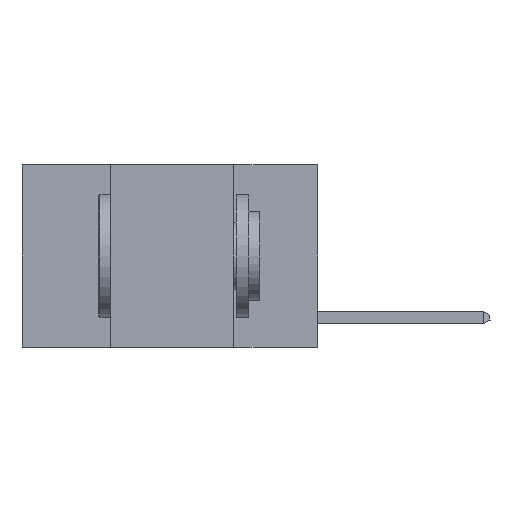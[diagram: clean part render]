
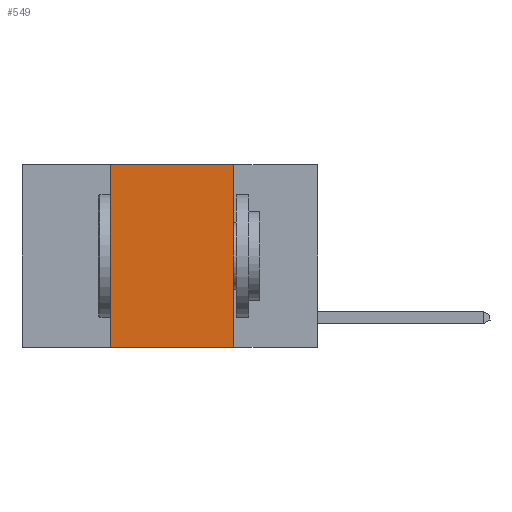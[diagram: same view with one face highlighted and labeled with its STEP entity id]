
A CAD part, left-side view. The second image highlights one B-rep face of the part: STEP entity #549.
In plain terms, the highlighted planar face has unit normal (-1, 0, 0).
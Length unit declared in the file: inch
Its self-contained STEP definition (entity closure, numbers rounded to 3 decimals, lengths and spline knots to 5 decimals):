
#181 = PLANE ( 'NONE',  #1054 ) ;
#549 = ADVANCED_FACE ( 'NONE', ( #6727 ), #181, .F. ) ;
#836 = ORIENTED_EDGE ( 'NONE', *, *, #5112, .F. ) ;
#945 = DIRECTION ( 'NONE',  ( 0., -1., 0. ) ) ;
#1054 = AXIS2_PLACEMENT_3D ( 'NONE', #6978, #3947, #5356 ) ;
#1161 = CARTESIAN_POINT ( 'NONE',  ( 0., 0.42, 0. ) ) ;
#2320 = CARTESIAN_POINT ( 'NONE',  ( 0., 0.17, 0. ) ) ;
#2432 = EDGE_LOOP ( 'NONE', ( #836, #7963, #5006, #6387 ) ) ;
#2466 = CARTESIAN_POINT ( 'NONE',  ( 0., 0.6, -0.37 ) ) ;
#2551 = DIRECTION ( 'NONE',  ( 0., -1., 0. ) ) ;
#2681 = DIRECTION ( 'NONE',  ( 0., 0., 1. ) ) ;
#2807 = VECTOR ( 'NONE', #8006, 39.37008 ) ;
#3322 = EDGE_CURVE ( 'NONE', #5777, #4982, #3911, .T. ) ;
#3737 = CARTESIAN_POINT ( 'NONE',  ( 0., 0.42, 0. ) ) ;
#3778 = LINE ( 'NONE', #2466, #9060 ) ;
#3911 = LINE ( 'NONE', #1161, #8978 ) ;
#3912 = VERTEX_POINT ( 'NONE', #6204 ) ;
#3947 = DIRECTION ( 'NONE',  ( 1., 0., 0. ) ) ;
#4150 = VECTOR ( 'NONE', #2551, 39.37008 ) ;
#4394 = LINE ( 'NONE', #6193, #4150 ) ;
#4504 = EDGE_CURVE ( 'NONE', #5777, #3912, #3778, .T. ) ;
#4982 = VERTEX_POINT ( 'NONE', #3737 ) ;
#5006 = ORIENTED_EDGE ( 'NONE', *, *, #3322, .F. ) ;
#5016 = CARTESIAN_POINT ( 'NONE',  ( 0., 0.42, -0.37 ) ) ;
#5112 = EDGE_CURVE ( 'NONE', #6689, #3912, #8434, .T. ) ;
#5356 = DIRECTION ( 'NONE',  ( 0., 0., -1. ) ) ;
#5777 = VERTEX_POINT ( 'NONE', #5016 ) ;
#6193 = CARTESIAN_POINT ( 'NONE',  ( 0., 0.6, 0. ) ) ;
#6204 = CARTESIAN_POINT ( 'NONE',  ( 0., 0.17, -0.37 ) ) ;
#6387 = ORIENTED_EDGE ( 'NONE', *, *, #4504, .T. ) ;
#6689 = VERTEX_POINT ( 'NONE', #9119 ) ;
#6727 = FACE_OUTER_BOUND ( 'NONE', #2432, .T. ) ;
#6978 = CARTESIAN_POINT ( 'NONE',  ( 0., 0.6, 0. ) ) ;
#7910 = EDGE_CURVE ( 'NONE', #4982, #6689, #4394, .T. ) ;
#7963 = ORIENTED_EDGE ( 'NONE', *, *, #7910, .F. ) ;
#8006 = DIRECTION ( 'NONE',  ( 0., 0., -1. ) ) ;
#8434 = LINE ( 'NONE', #2320, #2807 ) ;
#8978 = VECTOR ( 'NONE', #2681, 39.37008 ) ;
#9060 = VECTOR ( 'NONE', #945, 39.37008 ) ;
#9119 = CARTESIAN_POINT ( 'NONE',  ( 0., 0.17, 0. ) ) ;
